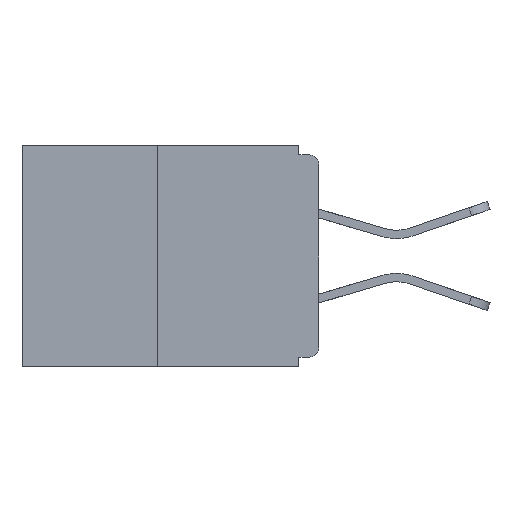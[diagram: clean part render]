
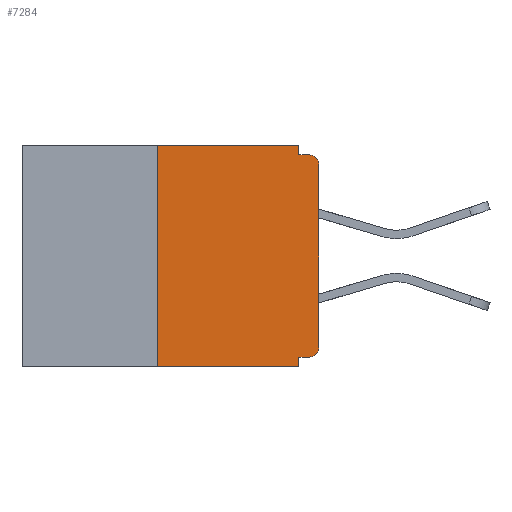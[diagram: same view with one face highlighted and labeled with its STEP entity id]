
A CAD part, left-side view. The second image highlights one B-rep face of the part: STEP entity #7284.
In plain terms, the highlighted planar face has unit normal (-1, 0, 0).
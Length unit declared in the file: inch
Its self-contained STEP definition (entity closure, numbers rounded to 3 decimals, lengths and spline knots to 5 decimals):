
#319 = CARTESIAN_POINT ( 'NONE',  ( 0., 0.031, -0.343 ) ) ;
#366 = VERTEX_POINT ( 'NONE', #2929 ) ;
#415 = EDGE_CURVE ( 'NONE', #2998, #2542, #4546, .T. ) ;
#624 = EDGE_CURVE ( 'NONE', #7135, #8424, #12105, .T. ) ;
#1378 = VECTOR ( 'NONE', #10190, 39.37008 ) ;
#1681 = LINE ( 'NONE', #8271, #1378 ) ;
#1769 = AXIS2_PLACEMENT_3D ( 'NONE', #9439, #11332, #11528 ) ;
#2131 = PLANE ( 'NONE',  #7205 ) ;
#2173 = LINE ( 'NONE', #10549, #3116 ) ;
#2189 = ORIENTED_EDGE ( 'NONE', *, *, #8209, .F. ) ;
#2472 = DIRECTION ( 'NONE',  ( 0., 0., -1. ) ) ;
#2542 = VERTEX_POINT ( 'NONE', #319 ) ;
#2790 = LINE ( 'NONE', #7449, #10900 ) ;
#2878 = CARTESIAN_POINT ( 'NONE',  ( 0., 0., -0.313 ) ) ;
#2909 = CARTESIAN_POINT ( 'NONE',  ( 0., 0.015, -0.328 ) ) ;
#2929 = CARTESIAN_POINT ( 'NONE',  ( 0., 0.031, -0.015 ) ) ;
#2937 = CARTESIAN_POINT ( 'NONE',  ( 0., 0.015, -0.015 ) ) ;
#2998 = VERTEX_POINT ( 'NONE', #8642 ) ;
#3007 = ORIENTED_EDGE ( 'NONE', *, *, #7529, .F. ) ;
#3116 = VECTOR ( 'NONE', #9420, 39.37008 ) ;
#3137 = VERTEX_POINT ( 'NONE', #11710 ) ;
#3296 = CARTESIAN_POINT ( 'NONE',  ( 0., 0., -0.328 ) ) ;
#3446 = VECTOR ( 'NONE', #4718, 39.37008 ) ;
#3684 = ORIENTED_EDGE ( 'NONE', *, *, #4252, .T. ) ;
#4252 = EDGE_CURVE ( 'NONE', #7135, #9748, #4774, .T. ) ;
#4546 = LINE ( 'NONE', #10048, #12723 ) ;
#4718 = DIRECTION ( 'NONE',  ( 0., 0., -1. ) ) ;
#4774 = CIRCLE ( 'NONE', #1769, 0.015 ) ;
#5076 = DIRECTION ( 'NONE',  ( 1., 0., 0. ) ) ;
#5162 = VERTEX_POINT ( 'NONE', #7881 ) ;
#5480 = ORIENTED_EDGE ( 'NONE', *, *, #9631, .F. ) ;
#5907 = CARTESIAN_POINT ( 'NONE',  ( 0., 0.25, 0. ) ) ;
#6064 = ORIENTED_EDGE ( 'NONE', *, *, #11890, .T. ) ;
#6726 = LINE ( 'NONE', #12710, #3446 ) ;
#7135 = VERTEX_POINT ( 'NONE', #2909 ) ;
#7205 = AXIS2_PLACEMENT_3D ( 'NONE', #11100, #5076, #11995 ) ;
#7284 = ADVANCED_FACE ( 'NONE', ( #11519 ), #2131, .F. ) ;
#7449 = CARTESIAN_POINT ( 'NONE',  ( 0., 0.031, 0. ) ) ;
#7529 = EDGE_CURVE ( 'NONE', #8424, #2542, #6726, .T. ) ;
#7573 = LINE ( 'NONE', #9224, #10774 ) ;
#7808 = CARTESIAN_POINT ( 'NONE',  ( 0., 0.015, -0.03 ) ) ;
#7881 = CARTESIAN_POINT ( 'NONE',  ( 0., 0., -0.03 ) ) ;
#7926 = VECTOR ( 'NONE', #12079, 39.37008 ) ;
#8209 = EDGE_CURVE ( 'NONE', #2998, #12760, #7573, .T. ) ;
#8240 = ORIENTED_EDGE ( 'NONE', *, *, #11467, .F. ) ;
#8271 = CARTESIAN_POINT ( 'NONE',  ( 0., 0., -0.015 ) ) ;
#8344 = DIRECTION ( 'NONE',  ( 0., 0., 1. ) ) ;
#8424 = VERTEX_POINT ( 'NONE', #10114 ) ;
#8468 = CIRCLE ( 'NONE', #10744, 0.015 ) ;
#8642 = CARTESIAN_POINT ( 'NONE',  ( 0., 0.25, -0.343 ) ) ;
#8782 = DIRECTION ( 'NONE',  ( -1., 0., 0. ) ) ;
#8867 = VECTOR ( 'NONE', #9193, 39.37008 ) ;
#9193 = DIRECTION ( 'NONE',  ( 0., 1., 0. ) ) ;
#9224 = CARTESIAN_POINT ( 'NONE',  ( 0., 0.25, 0. ) ) ;
#9287 = VERTEX_POINT ( 'NONE', #2937 ) ;
#9325 = LINE ( 'NONE', #11095, #7926 ) ;
#9404 = ORIENTED_EDGE ( 'NONE', *, *, #624, .F. ) ;
#9420 = DIRECTION ( 'NONE',  ( 0., -1., 0. ) ) ;
#9439 = CARTESIAN_POINT ( 'NONE',  ( 0., 0.015, -0.313 ) ) ;
#9605 = EDGE_LOOP ( 'NONE', ( #5480, #2189, #11399, #3007, #9404, #3684, #6064, #12773, #8240, #10848 ) ) ;
#9631 = EDGE_CURVE ( 'NONE', #12760, #3137, #2173, .T. ) ;
#9640 = EDGE_CURVE ( 'NONE', #3137, #366, #2790, .T. ) ;
#9651 = EDGE_CURVE ( 'NONE', #5162, #9287, #8468, .T. ) ;
#9730 = DIRECTION ( 'NONE',  ( 0., 0., -1. ) ) ;
#9748 = VERTEX_POINT ( 'NONE', #2878 ) ;
#10048 = CARTESIAN_POINT ( 'NONE',  ( 0., 0.46, -0.343 ) ) ;
#10114 = CARTESIAN_POINT ( 'NONE',  ( 0., 0.031, -0.328 ) ) ;
#10190 = DIRECTION ( 'NONE',  ( 0., -1., 0. ) ) ;
#10549 = CARTESIAN_POINT ( 'NONE',  ( 0., 0.46, 0. ) ) ;
#10744 = AXIS2_PLACEMENT_3D ( 'NONE', #7808, #8782, #9730 ) ;
#10774 = VECTOR ( 'NONE', #8344, 39.37008 ) ;
#10848 = ORIENTED_EDGE ( 'NONE', *, *, #9640, .F. ) ;
#10900 = VECTOR ( 'NONE', #2472, 39.37008 ) ;
#11095 = CARTESIAN_POINT ( 'NONE',  ( 0., 0., 0. ) ) ;
#11100 = CARTESIAN_POINT ( 'NONE',  ( 0., 0.46, 0. ) ) ;
#11332 = DIRECTION ( 'NONE',  ( -1., 0., 0. ) ) ;
#11399 = ORIENTED_EDGE ( 'NONE', *, *, #415, .T. ) ;
#11467 = EDGE_CURVE ( 'NONE', #366, #9287, #1681, .T. ) ;
#11519 = FACE_OUTER_BOUND ( 'NONE', #9605, .T. ) ;
#11528 = DIRECTION ( 'NONE',  ( 0., 0., -1. ) ) ;
#11710 = CARTESIAN_POINT ( 'NONE',  ( 0., 0.031, 0. ) ) ;
#11890 = EDGE_CURVE ( 'NONE', #9748, #5162, #9325, .T. ) ;
#11995 = DIRECTION ( 'NONE',  ( 0., 0., -1. ) ) ;
#12079 = DIRECTION ( 'NONE',  ( 0., 0., 1. ) ) ;
#12105 = LINE ( 'NONE', #3296, #8867 ) ;
#12710 = CARTESIAN_POINT ( 'NONE',  ( 0., 0.031, -0.343 ) ) ;
#12723 = VECTOR ( 'NONE', #12884, 39.37008 ) ;
#12760 = VERTEX_POINT ( 'NONE', #5907 ) ;
#12773 = ORIENTED_EDGE ( 'NONE', *, *, #9651, .T. ) ;
#12884 = DIRECTION ( 'NONE',  ( 0., -1., 0. ) ) ;
